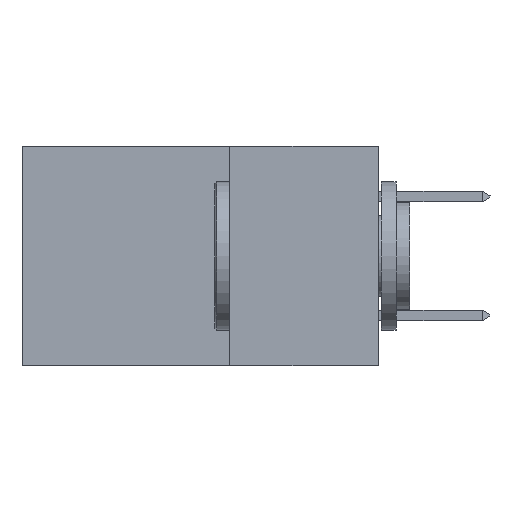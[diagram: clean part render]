
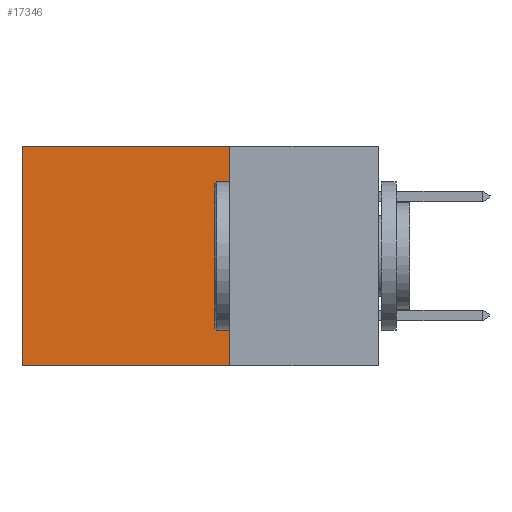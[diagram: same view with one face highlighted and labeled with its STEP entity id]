
A CAD part, left-side view. The second image highlights one B-rep face of the part: STEP entity #17346.
In plain terms, the highlighted planar face has unit normal (-1, 0, 0).
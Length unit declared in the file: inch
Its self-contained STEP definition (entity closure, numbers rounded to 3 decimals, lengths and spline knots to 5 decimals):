
#421 = EDGE_CURVE ( 'NONE', #8010, #25204, #6100, .T. ) ;
#2030 = VERTEX_POINT ( 'NONE', #15407 ) ;
#2537 = CARTESIAN_POINT ( 'NONE',  ( 0.2615, 0.25, -0.37 ) ) ;
#2867 = CARTESIAN_POINT ( 'NONE',  ( 0.2615, 0.25, -0.37 ) ) ;
#3305 = AXIS2_PLACEMENT_3D ( 'NONE', #2537, #10661, #18760 ) ;
#3400 = LINE ( 'NONE', #5270, #12938 ) ;
#3834 = CARTESIAN_POINT ( 'NONE',  ( 0.2615, 0.25, -0.37 ) ) ;
#4524 = PLANE ( 'NONE',  #3305 ) ;
#5270 = CARTESIAN_POINT ( 'NONE',  ( 0.2615, 0.25, 0. ) ) ;
#5690 = CARTESIAN_POINT ( 'NONE',  ( 0.2615, 0.25, -0.37 ) ) ;
#6100 = LINE ( 'NONE', #3834, #8946 ) ;
#6437 = CARTESIAN_POINT ( 'NONE',  ( 0.2615, 0.6, -0.37 ) ) ;
#8010 = VERTEX_POINT ( 'NONE', #19954 ) ;
#8143 = LINE ( 'NONE', #16244, #10110 ) ;
#8907 = ORIENTED_EDGE ( 'NONE', *, *, #17175, .T. ) ;
#8946 = VECTOR ( 'NONE', #18054, 39.37008 ) ;
#9080 = ORIENTED_EDGE ( 'NONE', *, *, #24110, .T. ) ;
#10110 = VECTOR ( 'NONE', #14244, 39.37008 ) ;
#10661 = DIRECTION ( 'NONE',  ( 1., 0., 0. ) ) ;
#12938 = VECTOR ( 'NONE', #21341, 39.37008 ) ;
#13897 = EDGE_CURVE ( 'NONE', #25204, #16652, #17147, .T. ) ;
#14215 = VECTOR ( 'NONE', #24010, 39.37008 ) ;
#14244 = DIRECTION ( 'NONE',  ( 0., 0., -1. ) ) ;
#15407 = CARTESIAN_POINT ( 'NONE',  ( 0.2615, 0.6, 0. ) ) ;
#16244 = CARTESIAN_POINT ( 'NONE',  ( 0.2615, 0.6, -0.37 ) ) ;
#16652 = VERTEX_POINT ( 'NONE', #6437 ) ;
#17147 = LINE ( 'NONE', #5690, #14215 ) ;
#17175 = EDGE_CURVE ( 'NONE', #2030, #16652, #8143, .T. ) ;
#17346 = ADVANCED_FACE ( 'NONE', ( #22755 ), #4524, .F. ) ;
#17423 = EDGE_LOOP ( 'NONE', ( #8907, #21746, #21419, #9080 ) ) ;
#18054 = DIRECTION ( 'NONE',  ( 0., 0., -1. ) ) ;
#18760 = DIRECTION ( 'NONE',  ( 0., 0., -1. ) ) ;
#19954 = CARTESIAN_POINT ( 'NONE',  ( 0.2615, 0.25, 0. ) ) ;
#21341 = DIRECTION ( 'NONE',  ( 0., 1., 0. ) ) ;
#21419 = ORIENTED_EDGE ( 'NONE', *, *, #421, .F. ) ;
#21746 = ORIENTED_EDGE ( 'NONE', *, *, #13897, .F. ) ;
#22755 = FACE_OUTER_BOUND ( 'NONE', #17423, .T. ) ;
#24010 = DIRECTION ( 'NONE',  ( 0., 1., 0. ) ) ;
#24110 = EDGE_CURVE ( 'NONE', #8010, #2030, #3400, .T. ) ;
#25204 = VERTEX_POINT ( 'NONE', #2867 ) ;
